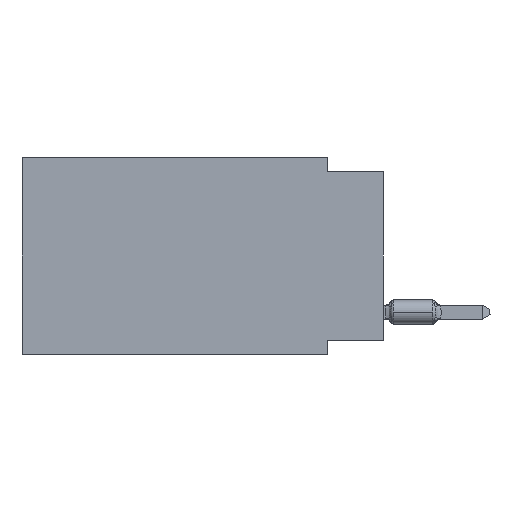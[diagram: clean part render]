
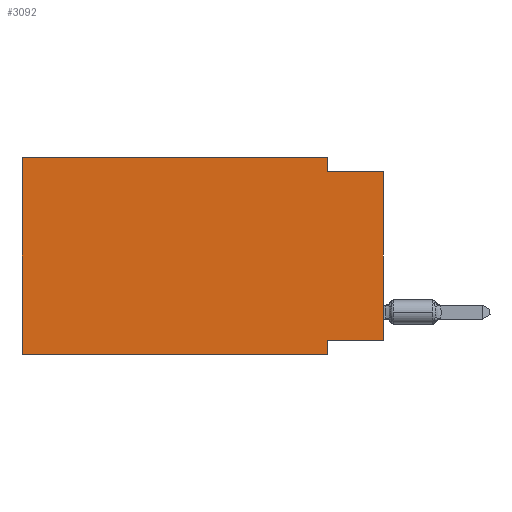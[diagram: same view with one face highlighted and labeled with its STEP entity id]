
A CAD part, left-side view. The second image highlights one B-rep face of the part: STEP entity #3092.
In plain terms, the highlighted planar face has unit normal (-1, 0, 0).
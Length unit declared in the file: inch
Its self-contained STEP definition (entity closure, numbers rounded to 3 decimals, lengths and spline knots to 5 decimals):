
#59 = LINE ( 'NONE', #12810, #6614 ) ;
#609 = VERTEX_POINT ( 'NONE', #13190 ) ;
#2121 = VERTEX_POINT ( 'NONE', #21010 ) ;
#2135 = DIRECTION ( 'NONE',  ( 0., 1., 0. ) ) ;
#2489 = CARTESIAN_POINT ( 'NONE',  ( 0., 0.645, -0.35 ) ) ;
#2491 = VERTEX_POINT ( 'NONE', #3581 ) ;
#2650 = EDGE_CURVE ( 'NONE', #15561, #609, #17184, .T. ) ;
#2779 = DIRECTION ( 'NONE',  ( 1., 0., 0. ) ) ;
#2848 = CARTESIAN_POINT ( 'NONE',  ( 0., 0.645, -0.35 ) ) ;
#2865 = DIRECTION ( 'NONE',  ( 0., 0., 1. ) ) ;
#2973 = CARTESIAN_POINT ( 'NONE',  ( 0., 0.645, 0. ) ) ;
#3092 = ADVANCED_FACE ( 'NONE', ( #13937 ), #14141, .F. ) ;
#3174 = DIRECTION ( 'NONE',  ( 0., 0., 1. ) ) ;
#3478 = ORIENTED_EDGE ( 'NONE', *, *, #12546, .F. ) ;
#3581 = CARTESIAN_POINT ( 'NONE',  ( 0., 0.645, 0. ) ) ;
#4390 = CARTESIAN_POINT ( 'NONE',  ( 0., 0.645, 0. ) ) ;
#4444 = VECTOR ( 'NONE', #3174, 39.37008 ) ;
#4657 = EDGE_CURVE ( 'NONE', #11290, #2121, #17143, .T. ) ;
#4707 = VECTOR ( 'NONE', #9029, 39.37008 ) ;
#4789 = CARTESIAN_POINT ( 'NONE',  ( 0., 0., 0. ) ) ;
#4872 = LINE ( 'NONE', #5580, #16584 ) ;
#4897 = VECTOR ( 'NONE', #2865, 39.37008 ) ;
#4980 = VECTOR ( 'NONE', #15427, 39.37008 ) ;
#5580 = CARTESIAN_POINT ( 'NONE',  ( 0., 0.645, 0. ) ) ;
#5738 = VERTEX_POINT ( 'NONE', #10010 ) ;
#6251 = CARTESIAN_POINT ( 'NONE',  ( 0., 0.1, -0.35 ) ) ;
#6614 = VECTOR ( 'NONE', #14638, 39.37008 ) ;
#6943 = EDGE_CURVE ( 'NONE', #11290, #8155, #19492, .T. ) ;
#7132 = AXIS2_PLACEMENT_3D ( 'NONE', #4390, #2779, #15755 ) ;
#7474 = LINE ( 'NONE', #2973, #4897 ) ;
#7698 = LINE ( 'NONE', #15640, #4980 ) ;
#8049 = ORIENTED_EDGE ( 'NONE', *, *, #9778, .F. ) ;
#8155 = VERTEX_POINT ( 'NONE', #15940 ) ;
#9029 = DIRECTION ( 'NONE',  ( 0., -1., 0. ) ) ;
#9360 = DIRECTION ( 'NONE',  ( 0., 0., -1. ) ) ;
#9778 = EDGE_CURVE ( 'NONE', #15561, #2491, #7474, .T. ) ;
#9821 = ORIENTED_EDGE ( 'NONE', *, *, #2650, .T. ) ;
#10010 = CARTESIAN_POINT ( 'NONE',  ( 0., 0.1, 0. ) ) ;
#10139 = ORIENTED_EDGE ( 'NONE', *, *, #4657, .F. ) ;
#10228 = ORIENTED_EDGE ( 'NONE', *, *, #12994, .F. ) ;
#10275 = EDGE_CURVE ( 'NONE', #5738, #12136, #59, .T. ) ;
#11290 = VERTEX_POINT ( 'NONE', #17763 ) ;
#12093 = VECTOR ( 'NONE', #2135, 39.37008 ) ;
#12136 = VERTEX_POINT ( 'NONE', #15769 ) ;
#12546 = EDGE_CURVE ( 'NONE', #12136, #8155, #7698, .T. ) ;
#12810 = CARTESIAN_POINT ( 'NONE',  ( 0., 0.1, 0. ) ) ;
#12994 = EDGE_CURVE ( 'NONE', #2121, #609, #20522, .T. ) ;
#13190 = CARTESIAN_POINT ( 'NONE',  ( 0., 0.1, -0.35 ) ) ;
#13269 = EDGE_CURVE ( 'NONE', #2491, #5738, #4872, .T. ) ;
#13828 = VECTOR ( 'NONE', #9360, 39.37008 ) ;
#13937 = FACE_OUTER_BOUND ( 'NONE', #17405, .T. ) ;
#14141 = PLANE ( 'NONE',  #7132 ) ;
#14638 = DIRECTION ( 'NONE',  ( 0., 0., -1. ) ) ;
#15427 = DIRECTION ( 'NONE',  ( 0., -1., 0. ) ) ;
#15561 = VERTEX_POINT ( 'NONE', #2848 ) ;
#15640 = CARTESIAN_POINT ( 'NONE',  ( 0., 0., -0.025 ) ) ;
#15755 = DIRECTION ( 'NONE',  ( 0., 0., -1. ) ) ;
#15769 = CARTESIAN_POINT ( 'NONE',  ( 0., 0.1, -0.025 ) ) ;
#15940 = CARTESIAN_POINT ( 'NONE',  ( 0., 0., -0.025 ) ) ;
#16584 = VECTOR ( 'NONE', #18674, 39.37008 ) ;
#17037 = CARTESIAN_POINT ( 'NONE',  ( 0., 0., -0.325 ) ) ;
#17143 = LINE ( 'NONE', #17037, #12093 ) ;
#17184 = LINE ( 'NONE', #2489, #4707 ) ;
#17208 = ORIENTED_EDGE ( 'NONE', *, *, #10275, .F. ) ;
#17405 = EDGE_LOOP ( 'NONE', ( #20532, #3478, #17208, #18737, #8049, #9821, #10228, #10139 ) ) ;
#17763 = CARTESIAN_POINT ( 'NONE',  ( 0., 0., -0.325 ) ) ;
#18674 = DIRECTION ( 'NONE',  ( 0., -1., 0. ) ) ;
#18737 = ORIENTED_EDGE ( 'NONE', *, *, #13269, .F. ) ;
#19492 = LINE ( 'NONE', #4789, #4444 ) ;
#20522 = LINE ( 'NONE', #6251, #13828 ) ;
#20532 = ORIENTED_EDGE ( 'NONE', *, *, #6943, .T. ) ;
#21010 = CARTESIAN_POINT ( 'NONE',  ( 0., 0.1, -0.325 ) ) ;
